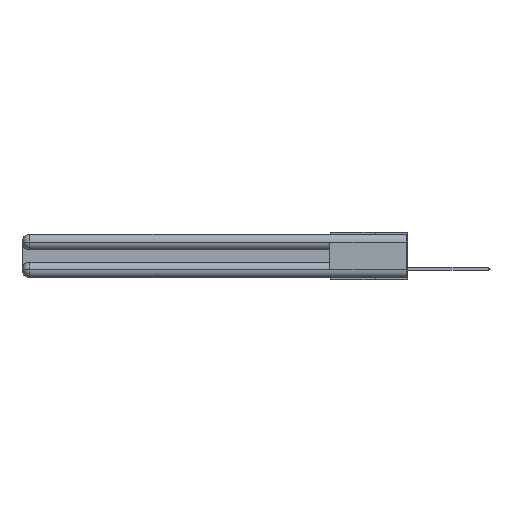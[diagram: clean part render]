
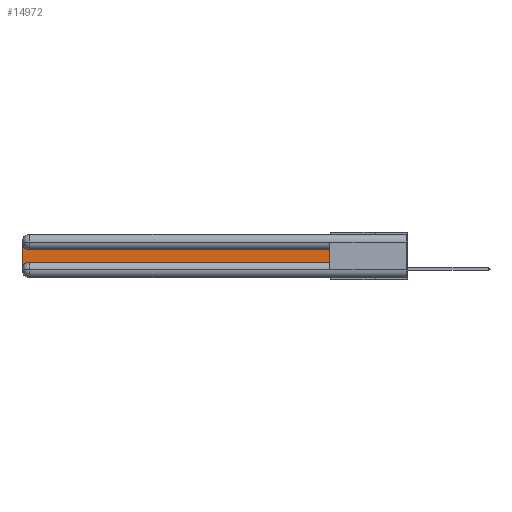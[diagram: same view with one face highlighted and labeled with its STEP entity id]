
A CAD part, left-side view. The second image highlights one B-rep face of the part: STEP entity #14972.
In plain terms, the highlighted planar face has unit normal (-1, 0, 0).
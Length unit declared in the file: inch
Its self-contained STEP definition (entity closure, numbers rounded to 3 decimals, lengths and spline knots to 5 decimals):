
#436 = VERTEX_POINT ( 'NONE', #26145 ) ;
#576 = VECTOR ( 'NONE', #26628, 39.37008 ) ;
#740 = VERTEX_POINT ( 'NONE', #22956 ) ;
#1015 = AXIS2_PLACEMENT_3D ( 'NONE', #17313, #17226, #10720 ) ;
#1459 = LINE ( 'NONE', #21983, #10365 ) ;
#2487 = EDGE_CURVE ( 'NONE', #740, #436, #13388, .T. ) ;
#2890 = ORIENTED_EDGE ( 'NONE', *, *, #27521, .T. ) ;
#3648 = LINE ( 'NONE', #21877, #18702 ) ;
#3860 = DIRECTION ( 'NONE',  ( 0., 0., -1. ) ) ;
#4683 = VECTOR ( 'NONE', #17649, 39.37008 ) ;
#4923 = AXIS2_PLACEMENT_3D ( 'NONE', #27757, #23751, #3860 ) ;
#5182 = CARTESIAN_POINT ( 'NONE',  ( 0.075, 0.6, -0.1225 ) ) ;
#6236 = CIRCLE ( 'NONE', #14872, 0.06 ) ;
#6514 = CARTESIAN_POINT ( 'NONE',  ( 0.075, 2.94, -0.2175 ) ) ;
#7151 = CARTESIAN_POINT ( 'NONE',  ( 0.075, 2.94, -0.2775 ) ) ;
#7796 = EDGE_CURVE ( 'NONE', #13797, #24310, #1459, .T. ) ;
#8752 = EDGE_LOOP ( 'NONE', ( #28025, #9166, #26629, #15159, #2890, #18876 ) ) ;
#8799 = DIRECTION ( 'NONE',  ( 0., 0., 1. ) ) ;
#9166 = ORIENTED_EDGE ( 'NONE', *, *, #2487, .T. ) ;
#9539 = EDGE_CURVE ( 'NONE', #10048, #13718, #6236, .T. ) ;
#10048 = VERTEX_POINT ( 'NONE', #13401 ) ;
#10365 = VECTOR ( 'NONE', #8799, 39.37008 ) ;
#10720 = DIRECTION ( 'NONE',  ( 0., 0., -1. ) ) ;
#11141 = CARTESIAN_POINT ( 'NONE',  ( 0.075, 0.6, -0.1225 ) ) ;
#11323 = CARTESIAN_POINT ( 'NONE',  ( 0.075, 3., -0.2175 ) ) ;
#13388 = CIRCLE ( 'NONE', #4923, 0.06 ) ;
#13401 = CARTESIAN_POINT ( 'NONE',  ( 0.075, 3., -0.2775 ) ) ;
#13718 = VERTEX_POINT ( 'NONE', #6514 ) ;
#13797 = VERTEX_POINT ( 'NONE', #22653 ) ;
#14872 = AXIS2_PLACEMENT_3D ( 'NONE', #7151, #24636, #16016 ) ;
#14972 = ADVANCED_FACE ( 'NONE', ( #21408 ), #21982, .F. ) ;
#15159 = ORIENTED_EDGE ( 'NONE', *, *, #9539, .T. ) ;
#15612 = EDGE_CURVE ( 'NONE', #24310, #740, #28286, .T. ) ;
#15754 = EDGE_CURVE ( 'NONE', #436, #10048, #25249, .T. ) ;
#15969 = DIRECTION ( 'NONE',  ( 0., -1., 0. ) ) ;
#16016 = DIRECTION ( 'NONE',  ( 0., 0., -1. ) ) ;
#17226 = DIRECTION ( 'NONE',  ( 1., 0., 0. ) ) ;
#17313 = CARTESIAN_POINT ( 'NONE',  ( 0.075, 3., -0.1225 ) ) ;
#17649 = DIRECTION ( 'NONE',  ( 0., 1., 0. ) ) ;
#18702 = VECTOR ( 'NONE', #15969, 39.37008 ) ;
#18876 = ORIENTED_EDGE ( 'NONE', *, *, #7796, .T. ) ;
#21408 = FACE_OUTER_BOUND ( 'NONE', #8752, .T. ) ;
#21877 = CARTESIAN_POINT ( 'NONE',  ( 0.075, 0.6, -0.2175 ) ) ;
#21982 = PLANE ( 'NONE',  #1015 ) ;
#21983 = CARTESIAN_POINT ( 'NONE',  ( 0.075, 0.6, -0.2175 ) ) ;
#22653 = CARTESIAN_POINT ( 'NONE',  ( 0.075, 0.6, -0.2175 ) ) ;
#22956 = CARTESIAN_POINT ( 'NONE',  ( 0.075, 2.94, -0.1225 ) ) ;
#23751 = DIRECTION ( 'NONE',  ( 1., 0., 0. ) ) ;
#24310 = VERTEX_POINT ( 'NONE', #5182 ) ;
#24636 = DIRECTION ( 'NONE',  ( 1., 0., 0. ) ) ;
#25249 = LINE ( 'NONE', #11323, #576 ) ;
#26145 = CARTESIAN_POINT ( 'NONE',  ( 0.075, 3., -0.0625 ) ) ;
#26628 = DIRECTION ( 'NONE',  ( 0., 0., -1. ) ) ;
#26629 = ORIENTED_EDGE ( 'NONE', *, *, #15754, .T. ) ;
#27521 = EDGE_CURVE ( 'NONE', #13718, #13797, #3648, .T. ) ;
#27757 = CARTESIAN_POINT ( 'NONE',  ( 0.075, 2.94, -0.0625 ) ) ;
#28025 = ORIENTED_EDGE ( 'NONE', *, *, #15612, .T. ) ;
#28286 = LINE ( 'NONE', #11141, #4683 ) ;
